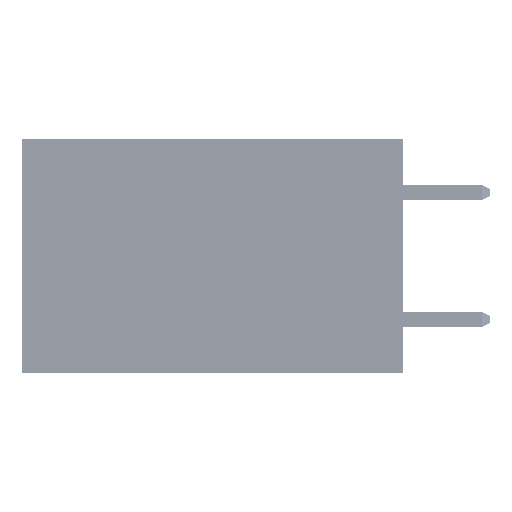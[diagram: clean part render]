
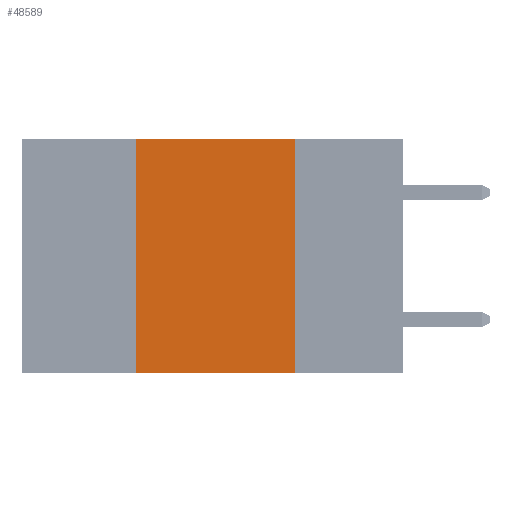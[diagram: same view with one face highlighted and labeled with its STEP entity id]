
A CAD part, left-side view. The second image highlights one B-rep face of the part: STEP entity #48589.
In plain terms, the highlighted planar face has unit normal (-1, 0, 0).
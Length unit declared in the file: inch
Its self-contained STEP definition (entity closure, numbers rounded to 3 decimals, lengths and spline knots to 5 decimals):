
#449 = EDGE_CURVE ( 'NONE', #27263, #48060, #7870, .T. ) ;
#1457 = ORIENTED_EDGE ( 'NONE', *, *, #30571, .T. ) ;
#1726 = DIRECTION ( 'NONE',  ( 0., -1., 0. ) ) ;
#4783 = CARTESIAN_POINT ( 'NONE',  ( 0., 0.42, -0.37 ) ) ;
#7339 = DIRECTION ( 'NONE',  ( 0., 0., 1. ) ) ;
#7481 = LINE ( 'NONE', #15538, #36220 ) ;
#7870 = LINE ( 'NONE', #32072, #25651 ) ;
#9581 = DIRECTION ( 'NONE',  ( 0., -1., 0. ) ) ;
#10394 = AXIS2_PLACEMENT_3D ( 'NONE', #16298, #13039, #25162 ) ;
#12991 = EDGE_LOOP ( 'NONE', ( #37411, #32884, #29637, #1457 ) ) ;
#13039 = DIRECTION ( 'NONE',  ( 1., 0., 0. ) ) ;
#13600 = LINE ( 'NONE', #46933, #21971 ) ;
#13947 = CARTESIAN_POINT ( 'NONE',  ( 0., 0.17, 0. ) ) ;
#15494 = FACE_OUTER_BOUND ( 'NONE', #12991, .T. ) ;
#15538 = CARTESIAN_POINT ( 'NONE',  ( 0., 0.17, 0. ) ) ;
#15985 = EDGE_CURVE ( 'NONE', #48060, #26776, #30764, .T. ) ;
#16298 = CARTESIAN_POINT ( 'NONE',  ( 0., 0.6, 0. ) ) ;
#21971 = VECTOR ( 'NONE', #9581, 39.37008 ) ;
#25162 = DIRECTION ( 'NONE',  ( 0., 0., -1. ) ) ;
#25651 = VECTOR ( 'NONE', #7339, 39.37008 ) ;
#26776 = VERTEX_POINT ( 'NONE', #13947 ) ;
#27263 = VERTEX_POINT ( 'NONE', #4783 ) ;
#29637 = ORIENTED_EDGE ( 'NONE', *, *, #449, .F. ) ;
#30571 = EDGE_CURVE ( 'NONE', #27263, #36156, #13600, .T. ) ;
#30764 = LINE ( 'NONE', #47147, #45492 ) ;
#32072 = CARTESIAN_POINT ( 'NONE',  ( 0., 0.42, 0. ) ) ;
#32751 = CARTESIAN_POINT ( 'NONE',  ( 0., 0.42, 0. ) ) ;
#32884 = ORIENTED_EDGE ( 'NONE', *, *, #15985, .F. ) ;
#33739 = PLANE ( 'NONE',  #10394 ) ;
#35740 = CARTESIAN_POINT ( 'NONE',  ( 0., 0.17, -0.37 ) ) ;
#36156 = VERTEX_POINT ( 'NONE', #35740 ) ;
#36220 = VECTOR ( 'NONE', #39728, 39.37008 ) ;
#37411 = ORIENTED_EDGE ( 'NONE', *, *, #45373, .F. ) ;
#39728 = DIRECTION ( 'NONE',  ( 0., 0., -1. ) ) ;
#45373 = EDGE_CURVE ( 'NONE', #26776, #36156, #7481, .T. ) ;
#45492 = VECTOR ( 'NONE', #1726, 39.37008 ) ;
#46933 = CARTESIAN_POINT ( 'NONE',  ( 0., 0.6, -0.37 ) ) ;
#47147 = CARTESIAN_POINT ( 'NONE',  ( 0., 0.6, 0. ) ) ;
#48060 = VERTEX_POINT ( 'NONE', #32751 ) ;
#48589 = ADVANCED_FACE ( 'NONE', ( #15494 ), #33739, .F. ) ;
